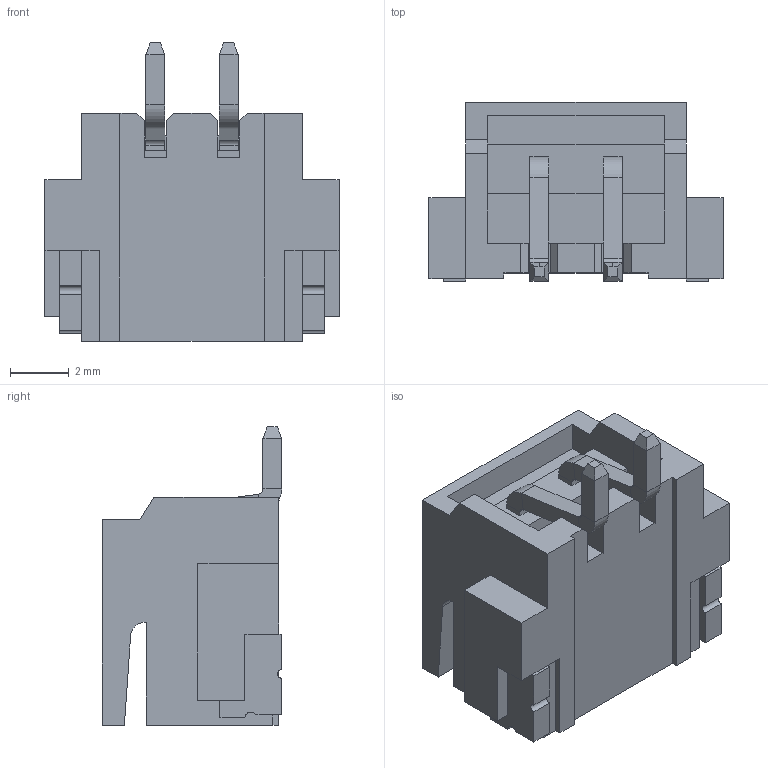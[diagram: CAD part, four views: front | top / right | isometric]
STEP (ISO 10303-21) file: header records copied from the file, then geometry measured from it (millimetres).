
FILE_DESCRIPTION (( 'STEP AP203' ), '1' );
FILE_NAME ('14K-502-418TAA1.STEP', '2024-02-22T13:13:20', ( '' ), ( '' ), 'SwSTEP 2.0', 'SolidWorks 2023', '' );
FILE_SCHEMA (( 'CONFIG_CONTROL_DESIGN' ));
Length unit declared in the file: millimetre
Products named in the file (3): 14K Series SMT Side Entry Insulator_502; 14K Series SMT Pin_Side Entry; 14K-502-418TAA1
Assembly tree (3 placements, depth 2):
  14K-502-418TAA1
    14K Series SMT Side Entry Insulator_502
    14K Series SMT Pin_Side Entry  x2
Bounding box: 10 x 6.1 x 10.15 mm (x, y, z)
Volume: 184.6 mm3; surface area: 534.3 mm2
Topology: 3 solids, 3 shells, 185 faces, 477 edges, 298 vertices
Faces by surface type: plane 166, cylinder 19
Entity records: 5012 total; most frequent: CARTESIAN_POINT 832, ORIENTED_EDGE 822, DIRECTION 759, EDGE_CURVE 411, LINE 381, VECTOR 381, VERTEX_POINT 262, AXIS2_PLACEMENT_3D 189
